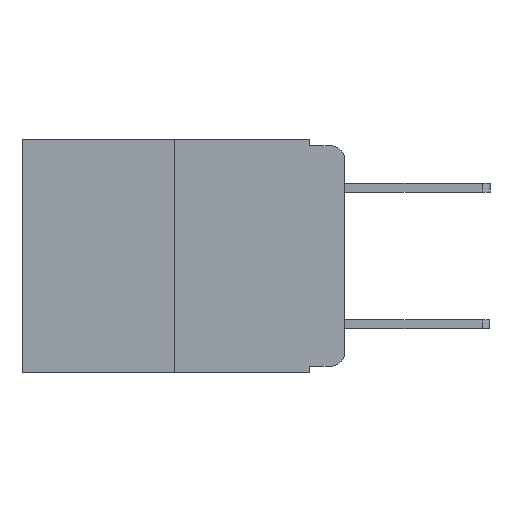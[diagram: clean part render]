
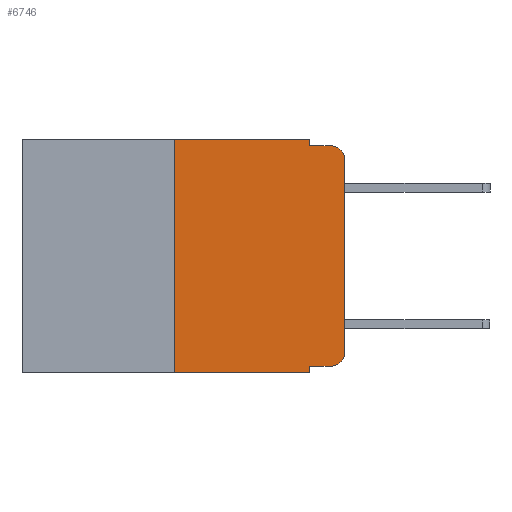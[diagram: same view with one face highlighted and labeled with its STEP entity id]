
A CAD part, left-side view. The second image highlights one B-rep face of the part: STEP entity #6746.
In plain terms, the highlighted planar face has unit normal (-1, 0, 0).
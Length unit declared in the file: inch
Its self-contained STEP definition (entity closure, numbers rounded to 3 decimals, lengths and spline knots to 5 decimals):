
#26 = CARTESIAN_POINT ( 'NONE',  ( 0., 0., 0. ) ) ;
#28 = VECTOR ( 'NONE', #6050, 39.37008 ) ;
#122 = EDGE_CURVE ( 'NONE', #756, #3076, #2206, .T. ) ;
#439 = DIRECTION ( 'NONE',  ( 0., 0., 1. ) ) ;
#592 = LINE ( 'NONE', #5470, #8892 ) ;
#756 = VERTEX_POINT ( 'NONE', #5301 ) ;
#872 = LINE ( 'NONE', #1317, #7112 ) ;
#1094 = CIRCLE ( 'NONE', #9027, 0.02 ) ;
#1125 = CARTESIAN_POINT ( 'NONE',  ( 0., 0.473, 0. ) ) ;
#1317 = CARTESIAN_POINT ( 'NONE',  ( 0., 0.25, 0. ) ) ;
#1534 = EDGE_LOOP ( 'NONE', ( #7958, #8201, #1883, #6392, #8442, #4548, #6894, #8924, #2723, #7132 ) ) ;
#1602 = VECTOR ( 'NONE', #5010, 39.37008 ) ;
#1691 = EDGE_CURVE ( 'NONE', #6985, #6813, #10209, .T. ) ;
#1883 = ORIENTED_EDGE ( 'NONE', *, *, #9226, .F. ) ;
#2071 = DIRECTION ( 'NONE',  ( 0., 0., -1. ) ) ;
#2206 = LINE ( 'NONE', #26, #6435 ) ;
#2402 = LINE ( 'NONE', #5252, #28 ) ;
#2468 = CARTESIAN_POINT ( 'NONE',  ( 0., 0.051, 0. ) ) ;
#2618 = CARTESIAN_POINT ( 'NONE',  ( 0., 0., -0.03 ) ) ;
#2624 = VERTEX_POINT ( 'NONE', #10258 ) ;
#2723 = ORIENTED_EDGE ( 'NONE', *, *, #7177, .T. ) ;
#2759 = DIRECTION ( 'NONE',  ( 0., 0., 1. ) ) ;
#3076 = VERTEX_POINT ( 'NONE', #2618 ) ;
#3094 = VECTOR ( 'NONE', #3545, 39.37008 ) ;
#3513 = CARTESIAN_POINT ( 'NONE',  ( 0., 0.051, -0.01 ) ) ;
#3545 = DIRECTION ( 'NONE',  ( 0., -1., 0. ) ) ;
#3553 = CARTESIAN_POINT ( 'NONE',  ( 0., 0.051, -0.333 ) ) ;
#3653 = EDGE_CURVE ( 'NONE', #10188, #2624, #6975, .T. ) ;
#3759 = CARTESIAN_POINT ( 'NONE',  ( 0., 0.02, -0.313 ) ) ;
#3773 = VERTEX_POINT ( 'NONE', #7901 ) ;
#3797 = DIRECTION ( 'NONE',  ( 0., 0., -1. ) ) ;
#4192 = CARTESIAN_POINT ( 'NONE',  ( 0., 0.02, -0.03 ) ) ;
#4264 = VECTOR ( 'NONE', #9119, 39.37008 ) ;
#4512 = AXIS2_PLACEMENT_3D ( 'NONE', #1125, #7085, #2071 ) ;
#4548 = ORIENTED_EDGE ( 'NONE', *, *, #8187, .F. ) ;
#4649 = DIRECTION ( 'NONE',  ( 0., 0., -1. ) ) ;
#4772 = CARTESIAN_POINT ( 'NONE',  ( 0., 0.25, 0. ) ) ;
#5010 = DIRECTION ( 'NONE',  ( 0., -1., 0. ) ) ;
#5032 = DIRECTION ( 'NONE',  ( 0., 0., -1. ) ) ;
#5252 = CARTESIAN_POINT ( 'NONE',  ( 0., 0.051, -0.01 ) ) ;
#5301 = CARTESIAN_POINT ( 'NONE',  ( 0., 0., -0.313 ) ) ;
#5470 = CARTESIAN_POINT ( 'NONE',  ( 0., 0.051, 0. ) ) ;
#5488 = PLANE ( 'NONE',  #4512 ) ;
#5706 = CARTESIAN_POINT ( 'NONE',  ( 0., 0.051, -0.333 ) ) ;
#6050 = DIRECTION ( 'NONE',  ( 0., -1., 0. ) ) ;
#6172 = VERTEX_POINT ( 'NONE', #5706 ) ;
#6392 = ORIENTED_EDGE ( 'NONE', *, *, #8689, .F. ) ;
#6435 = VECTOR ( 'NONE', #2759, 39.37008 ) ;
#6649 = EDGE_CURVE ( 'NONE', #8939, #756, #6899, .T. ) ;
#6746 = ADVANCED_FACE ( 'NONE', ( #10213 ), #5488, .F. ) ;
#6813 = VERTEX_POINT ( 'NONE', #9446 ) ;
#6880 = VECTOR ( 'NONE', #9753, 39.37008 ) ;
#6894 = ORIENTED_EDGE ( 'NONE', *, *, #1691, .T. ) ;
#6899 = CIRCLE ( 'NONE', #10398, 0.02 ) ;
#6975 = LINE ( 'NONE', #8339, #3094 ) ;
#6985 = VERTEX_POINT ( 'NONE', #7404 ) ;
#7085 = DIRECTION ( 'NONE',  ( 1., 0., 0. ) ) ;
#7112 = VECTOR ( 'NONE', #439, 39.37008 ) ;
#7132 = ORIENTED_EDGE ( 'NONE', *, *, #6649, .T. ) ;
#7177 = EDGE_CURVE ( 'NONE', #6172, #8939, #8437, .T. ) ;
#7404 = CARTESIAN_POINT ( 'NONE',  ( 0., 0.25, -0.343 ) ) ;
#7694 = EDGE_CURVE ( 'NONE', #6172, #6813, #8914, .T. ) ;
#7901 = CARTESIAN_POINT ( 'NONE',  ( 0., 0.02, -0.01 ) ) ;
#7958 = ORIENTED_EDGE ( 'NONE', *, *, #122, .T. ) ;
#8187 = EDGE_CURVE ( 'NONE', #6985, #10188, #872, .T. ) ;
#8201 = ORIENTED_EDGE ( 'NONE', *, *, #9725, .T. ) ;
#8339 = CARTESIAN_POINT ( 'NONE',  ( 0., 0.473, 0. ) ) ;
#8437 = LINE ( 'NONE', #3553, #4264 ) ;
#8442 = ORIENTED_EDGE ( 'NONE', *, *, #3653, .F. ) ;
#8453 = VERTEX_POINT ( 'NONE', #3513 ) ;
#8689 = EDGE_CURVE ( 'NONE', #2624, #8453, #592, .T. ) ;
#8852 = CARTESIAN_POINT ( 'NONE',  ( 0., 0.473, -0.343 ) ) ;
#8892 = VECTOR ( 'NONE', #3797, 39.37008 ) ;
#8914 = LINE ( 'NONE', #2468, #6880 ) ;
#8924 = ORIENTED_EDGE ( 'NONE', *, *, #7694, .F. ) ;
#8939 = VERTEX_POINT ( 'NONE', #10301 ) ;
#9027 = AXIS2_PLACEMENT_3D ( 'NONE', #4192, #9649, #5032 ) ;
#9119 = DIRECTION ( 'NONE',  ( 0., -1., 0. ) ) ;
#9226 = EDGE_CURVE ( 'NONE', #8453, #3773, #2402, .T. ) ;
#9288 = DIRECTION ( 'NONE',  ( -1., 0., 0. ) ) ;
#9446 = CARTESIAN_POINT ( 'NONE',  ( 0., 0.051, -0.343 ) ) ;
#9649 = DIRECTION ( 'NONE',  ( -1., 0., 0. ) ) ;
#9725 = EDGE_CURVE ( 'NONE', #3076, #3773, #1094, .T. ) ;
#9753 = DIRECTION ( 'NONE',  ( 0., 0., -1. ) ) ;
#10188 = VERTEX_POINT ( 'NONE', #4772 ) ;
#10209 = LINE ( 'NONE', #8852, #1602 ) ;
#10213 = FACE_OUTER_BOUND ( 'NONE', #1534, .T. ) ;
#10258 = CARTESIAN_POINT ( 'NONE',  ( 0., 0.051, 0. ) ) ;
#10301 = CARTESIAN_POINT ( 'NONE',  ( 0., 0.02, -0.333 ) ) ;
#10398 = AXIS2_PLACEMENT_3D ( 'NONE', #3759, #9288, #4649 ) ;
